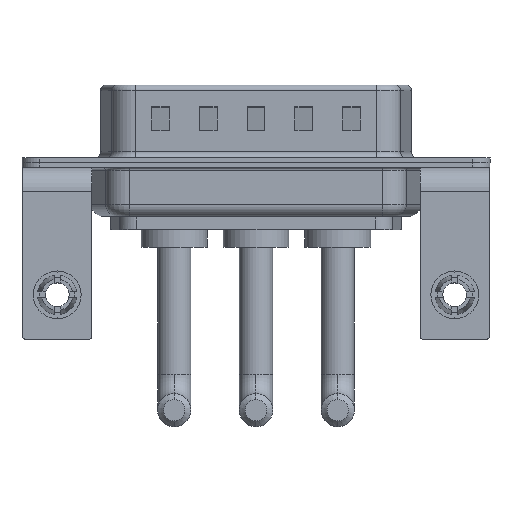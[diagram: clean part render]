
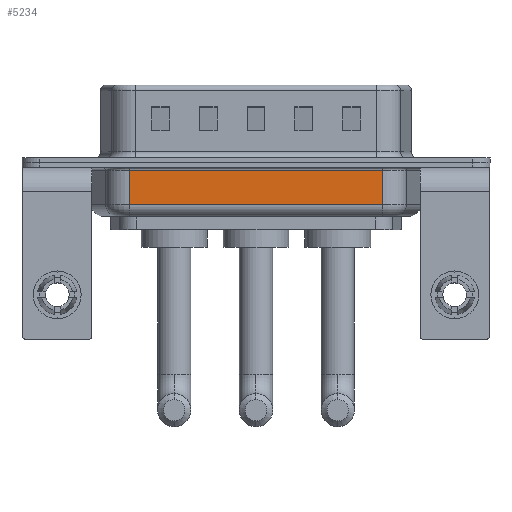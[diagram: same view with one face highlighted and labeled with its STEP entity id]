
A CAD part, front view. The second image highlights one B-rep face of the part: STEP entity #5234.
In plain terms, the highlighted planar face has unit normal (0, -1, 0).
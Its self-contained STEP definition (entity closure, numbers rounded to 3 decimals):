
#226 = DIRECTION ( 'NONE',  ( 0., 1., 0. ) ) ;
#471 = CARTESIAN_POINT ( 'NONE',  ( 6.031, -5.35, -0.65 ) ) ;
#519 = CARTESIAN_POINT ( 'NONE',  ( 27.269, -5.35, -0.65 ) ) ;
#591 = PLANE ( 'NONE',  #11477 ) ;
#2362 = ORIENTED_EDGE ( 'NONE', *, *, #16386, .T. ) ;
#2728 = CARTESIAN_POINT ( 'NONE',  ( 6.031, -5.35, -3.5 ) ) ;
#3450 = DIRECTION ( 'NONE',  ( 0., 0., 1. ) ) ;
#3672 = LINE ( 'NONE', #13441, #13109 ) ;
#3796 = CARTESIAN_POINT ( 'NONE',  ( 6.031, -5.35, -0.65 ) ) ;
#3887 = EDGE_CURVE ( 'NONE', #10637, #14742, #15464, .T. ) ;
#4237 = VECTOR ( 'NONE', #3450, 1000. ) ;
#5084 = EDGE_CURVE ( 'NONE', #14286, #8136, #16235, .T. ) ;
#5234 = ADVANCED_FACE ( 'NONE', ( #13245 ), #591, .F. ) ;
#6242 = CARTESIAN_POINT ( 'NONE',  ( 6.031, -5.35, -4.5 ) ) ;
#8136 = VERTEX_POINT ( 'NONE', #471 ) ;
#8453 = CARTESIAN_POINT ( 'NONE',  ( 6.031, -5.35, -3.5 ) ) ;
#9100 = DIRECTION ( 'NONE',  ( 0., 0., 1. ) ) ;
#9707 = VECTOR ( 'NONE', #14863, 1000. ) ;
#9746 = VECTOR ( 'NONE', #14176, 1000. ) ;
#10467 = EDGE_LOOP ( 'NONE', ( #14382, #14034, #2362, #12514 ) ) ;
#10637 = VERTEX_POINT ( 'NONE', #2728 ) ;
#11477 = AXIS2_PLACEMENT_3D ( 'NONE', #6242, #226, #17308 ) ;
#11933 = CARTESIAN_POINT ( 'NONE',  ( 6.031, -5.35, -4.5 ) ) ;
#12304 = CARTESIAN_POINT ( 'NONE',  ( 27.269, -5.35, -3.5 ) ) ;
#12514 = ORIENTED_EDGE ( 'NONE', *, *, #5084, .T. ) ;
#13109 = VECTOR ( 'NONE', #9100, 1000. ) ;
#13245 = FACE_OUTER_BOUND ( 'NONE', #10467, .T. ) ;
#13441 = CARTESIAN_POINT ( 'NONE',  ( 27.269, -5.35, -4.5 ) ) ;
#13468 = EDGE_CURVE ( 'NONE', #10637, #8136, #17645, .T. ) ;
#14034 = ORIENTED_EDGE ( 'NONE', *, *, #3887, .T. ) ;
#14176 = DIRECTION ( 'NONE',  ( 1., 0., 0. ) ) ;
#14286 = VERTEX_POINT ( 'NONE', #519 ) ;
#14382 = ORIENTED_EDGE ( 'NONE', *, *, #13468, .F. ) ;
#14742 = VERTEX_POINT ( 'NONE', #12304 ) ;
#14863 = DIRECTION ( 'NONE',  ( -1., 0., 0. ) ) ;
#15464 = LINE ( 'NONE', #8453, #9746 ) ;
#16235 = LINE ( 'NONE', #3796, #9707 ) ;
#16386 = EDGE_CURVE ( 'NONE', #14742, #14286, #3672, .T. ) ;
#17308 = DIRECTION ( 'NONE',  ( 0., 0., 1. ) ) ;
#17645 = LINE ( 'NONE', #11933, #4237 ) ;
